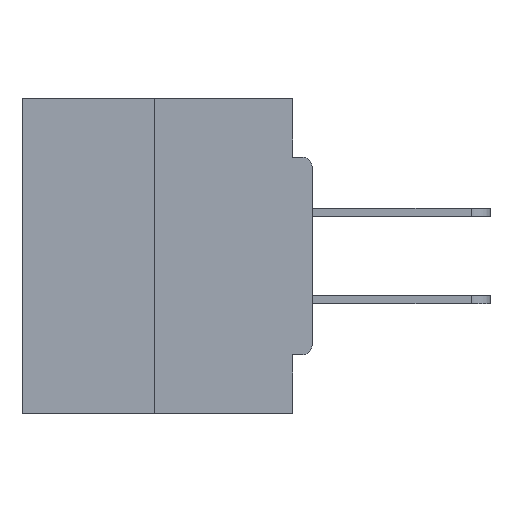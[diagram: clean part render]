
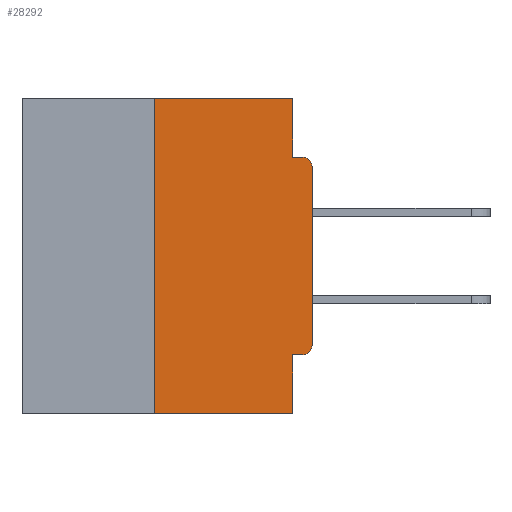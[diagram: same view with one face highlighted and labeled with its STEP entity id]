
A CAD part, left-side view. The second image highlights one B-rep face of the part: STEP entity #28292.
In plain terms, the highlighted planar face has unit normal (-1, 0, 0).
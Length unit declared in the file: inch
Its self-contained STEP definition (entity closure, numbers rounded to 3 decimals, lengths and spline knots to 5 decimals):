
#783 = EDGE_LOOP ( 'NONE', ( #16302, #25667, #12480, #24317, #31525, #30361, #8271, #13884, #14815, #23343 ) ) ;
#840 = VERTEX_POINT ( 'NONE', #11197 ) ;
#1007 = LINE ( 'NONE', #26887, #4914 ) ;
#1829 = VECTOR ( 'NONE', #31224, 39.37008 ) ;
#2219 = AXIS2_PLACEMENT_3D ( 'NONE', #23062, #10705, #23382 ) ;
#2584 = DIRECTION ( 'NONE',  ( 0., -1., 0. ) ) ;
#3182 = VERTEX_POINT ( 'NONE', #23861 ) ;
#3545 = PLANE ( 'NONE',  #24881 ) ;
#3982 = LINE ( 'NONE', #31074, #18084 ) ;
#4148 = VERTEX_POINT ( 'NONE', #20349 ) ;
#4258 = CARTESIAN_POINT ( 'NONE',  ( 0., 0.25, -0.5 ) ) ;
#4746 = EDGE_CURVE ( 'NONE', #12189, #30160, #1007, .T. ) ;
#4914 = VECTOR ( 'NONE', #14339, 39.37008 ) ;
#6550 = DIRECTION ( 'NONE',  ( -1., 0., 0. ) ) ;
#8047 = EDGE_CURVE ( 'NONE', #30160, #14760, #20315, .T. ) ;
#8271 = ORIENTED_EDGE ( 'NONE', *, *, #4746, .T. ) ;
#8512 = DIRECTION ( 'NONE',  ( 0., -1., 0. ) ) ;
#9078 = EDGE_CURVE ( 'NONE', #3182, #4148, #14338, .T. ) ;
#9264 = CARTESIAN_POINT ( 'NONE',  ( 0., 0.015, -0.0935 ) ) ;
#9615 = DIRECTION ( 'NONE',  ( 0., -1., 0. ) ) ;
#9986 = EDGE_CURVE ( 'NONE', #18339, #4148, #20571, .T. ) ;
#10387 = DIRECTION ( 'NONE',  ( 0., 0., -1. ) ) ;
#10705 = DIRECTION ( 'NONE',  ( -1., 0., 0. ) ) ;
#10765 = CARTESIAN_POINT ( 'NONE',  ( 0., 0., -0.4065 ) ) ;
#11197 = CARTESIAN_POINT ( 'NONE',  ( 0., 0.015, -0.4065 ) ) ;
#11403 = LINE ( 'NONE', #25768, #30682 ) ;
#11942 = CARTESIAN_POINT ( 'NONE',  ( 0., 0.46, -0.5 ) ) ;
#12012 = CIRCLE ( 'NONE', #2219, 0.015 ) ;
#12189 = VERTEX_POINT ( 'NONE', #25960 ) ;
#12480 = ORIENTED_EDGE ( 'NONE', *, *, #9986, .T. ) ;
#12503 = CARTESIAN_POINT ( 'NONE',  ( 0., 0.25, 0. ) ) ;
#13083 = DIRECTION ( 'NONE',  ( 0., 1., 0. ) ) ;
#13429 = CARTESIAN_POINT ( 'NONE',  ( 0., 0.031, -0.5 ) ) ;
#13884 = ORIENTED_EDGE ( 'NONE', *, *, #8047, .T. ) ;
#13890 = EDGE_CURVE ( 'NONE', #18339, #16369, #25980, .T. ) ;
#14102 = CARTESIAN_POINT ( 'NONE',  ( 0., 0.031, 0. ) ) ;
#14163 = EDGE_CURVE ( 'NONE', #17791, #14760, #25559, .T. ) ;
#14338 = LINE ( 'NONE', #13429, #1829 ) ;
#14339 = DIRECTION ( 'NONE',  ( 0., 0., 1. ) ) ;
#14688 = EDGE_CURVE ( 'NONE', #16369, #22529, #3982, .T. ) ;
#14760 = VERTEX_POINT ( 'NONE', #9264 ) ;
#14776 = DIRECTION ( 'NONE',  ( 0., 0., 1. ) ) ;
#14815 = ORIENTED_EDGE ( 'NONE', *, *, #14163, .F. ) ;
#15732 = VECTOR ( 'NONE', #2584, 39.37008 ) ;
#16302 = ORIENTED_EDGE ( 'NONE', *, *, #14688, .F. ) ;
#16369 = VERTEX_POINT ( 'NONE', #12503 ) ;
#17346 = CARTESIAN_POINT ( 'NONE',  ( 0., 0.25, 0. ) ) ;
#17791 = VERTEX_POINT ( 'NONE', #31633 ) ;
#18084 = VECTOR ( 'NONE', #8512, 39.37008 ) ;
#18339 = VERTEX_POINT ( 'NONE', #4258 ) ;
#18973 = DIRECTION ( 'NONE',  ( 1., 0., 0. ) ) ;
#20315 = CIRCLE ( 'NONE', #22144, 0.015 ) ;
#20349 = CARTESIAN_POINT ( 'NONE',  ( 0., 0.031, -0.5 ) ) ;
#20571 = LINE ( 'NONE', #11942, #30782 ) ;
#21778 = EDGE_CURVE ( 'NONE', #840, #3182, #26815, .T. ) ;
#21803 = CARTESIAN_POINT ( 'NONE',  ( 0., 0.015, -0.1085 ) ) ;
#22144 = AXIS2_PLACEMENT_3D ( 'NONE', #21803, #6550, #24141 ) ;
#22529 = VERTEX_POINT ( 'NONE', #14102 ) ;
#22917 = VECTOR ( 'NONE', #13083, 39.37008 ) ;
#23015 = CARTESIAN_POINT ( 'NONE',  ( 0., 0., -0.0935 ) ) ;
#23062 = CARTESIAN_POINT ( 'NONE',  ( 0., 0.015, -0.3915 ) ) ;
#23343 = ORIENTED_EDGE ( 'NONE', *, *, #27360, .F. ) ;
#23382 = DIRECTION ( 'NONE',  ( 0., 0., -1. ) ) ;
#23704 = DIRECTION ( 'NONE',  ( 0., 0., -1. ) ) ;
#23861 = CARTESIAN_POINT ( 'NONE',  ( 0., 0.031, -0.4065 ) ) ;
#24035 = CARTESIAN_POINT ( 'NONE',  ( 0., 0.46, 0. ) ) ;
#24141 = DIRECTION ( 'NONE',  ( 0., 0., -1. ) ) ;
#24317 = ORIENTED_EDGE ( 'NONE', *, *, #9078, .F. ) ;
#24881 = AXIS2_PLACEMENT_3D ( 'NONE', #24035, #18973, #23704 ) ;
#25559 = LINE ( 'NONE', #23015, #15732 ) ;
#25667 = ORIENTED_EDGE ( 'NONE', *, *, #13890, .F. ) ;
#25768 = CARTESIAN_POINT ( 'NONE',  ( 0., 0.031, 0. ) ) ;
#25960 = CARTESIAN_POINT ( 'NONE',  ( 0., 0., -0.3915 ) ) ;
#25980 = LINE ( 'NONE', #17346, #30720 ) ;
#26815 = LINE ( 'NONE', #10765, #22917 ) ;
#26887 = CARTESIAN_POINT ( 'NONE',  ( 0., 0., 0. ) ) ;
#27360 = EDGE_CURVE ( 'NONE', #22529, #17791, #11403, .T. ) ;
#27740 = CARTESIAN_POINT ( 'NONE',  ( 0., 0., -0.1085 ) ) ;
#28292 = ADVANCED_FACE ( 'NONE', ( #31396 ), #3545, .F. ) ;
#29773 = EDGE_CURVE ( 'NONE', #840, #12189, #12012, .T. ) ;
#30160 = VERTEX_POINT ( 'NONE', #27740 ) ;
#30361 = ORIENTED_EDGE ( 'NONE', *, *, #29773, .T. ) ;
#30682 = VECTOR ( 'NONE', #10387, 39.37008 ) ;
#30720 = VECTOR ( 'NONE', #14776, 39.37008 ) ;
#30782 = VECTOR ( 'NONE', #9615, 39.37008 ) ;
#31074 = CARTESIAN_POINT ( 'NONE',  ( 0., 0.46, 0. ) ) ;
#31224 = DIRECTION ( 'NONE',  ( 0., 0., -1. ) ) ;
#31396 = FACE_OUTER_BOUND ( 'NONE', #783, .T. ) ;
#31525 = ORIENTED_EDGE ( 'NONE', *, *, #21778, .F. ) ;
#31633 = CARTESIAN_POINT ( 'NONE',  ( 0., 0.031, -0.0935 ) ) ;
